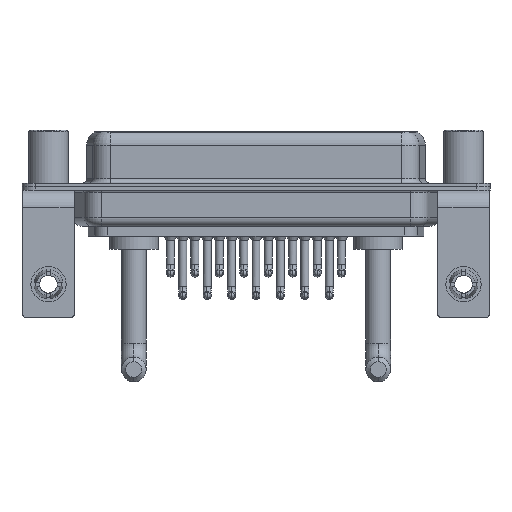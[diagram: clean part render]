
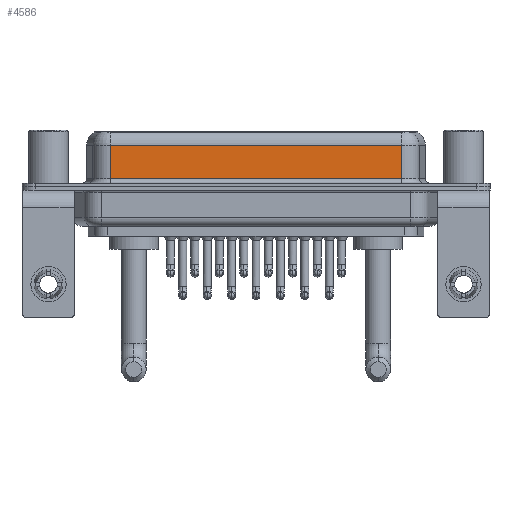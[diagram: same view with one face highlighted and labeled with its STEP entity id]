
A CAD part, front view. The second image highlights one B-rep face of the part: STEP entity #4586.
In plain terms, the highlighted planar face has unit normal (0, -1, 0).
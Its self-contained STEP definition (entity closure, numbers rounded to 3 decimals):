
#231 = VECTOR ( 'NONE', #15734, 1000. ) ;
#411 = LINE ( 'NONE', #7997, #231 ) ;
#575 = LINE ( 'NONE', #22193, #4274 ) ;
#616 = DIRECTION ( 'NONE',  ( 0., 0., -1. ) ) ;
#839 = VERTEX_POINT ( 'NONE', #9190 ) ;
#2372 = VERTEX_POINT ( 'NONE', #9619 ) ;
#2767 = VERTEX_POINT ( 'NONE', #7448 ) ;
#2975 = VECTOR ( 'NONE', #23240, 1000. ) ;
#3736 = CARTESIAN_POINT ( 'NONE',  ( 7.013, -3.95, 0.9 ) ) ;
#3805 = ORIENTED_EDGE ( 'NONE', *, *, #18545, .T. ) ;
#4130 = EDGE_LOOP ( 'NONE', ( #24198, #3805, #7274, #6062 ) ) ;
#4274 = VECTOR ( 'NONE', #20297, 1000. ) ;
#4586 = ADVANCED_FACE ( 'NONE', ( #7038 ), #23507, .F. ) ;
#5246 = EDGE_CURVE ( 'NONE', #10804, #2372, #575, .T. ) ;
#6062 = ORIENTED_EDGE ( 'NONE', *, *, #5246, .T. ) ;
#6183 = LINE ( 'NONE', #21618, #18519 ) ;
#7038 = FACE_OUTER_BOUND ( 'NONE', #4130, .T. ) ;
#7274 = ORIENTED_EDGE ( 'NONE', *, *, #21996, .T. ) ;
#7448 = CARTESIAN_POINT ( 'NONE',  ( 7.013, -3.95, 4.65 ) ) ;
#7997 = CARTESIAN_POINT ( 'NONE',  ( 40.037, -3.95, 4.65 ) ) ;
#8340 = DIRECTION ( 'NONE',  ( 0., 0., 1. ) ) ;
#8921 = CARTESIAN_POINT ( 'NONE',  ( 40.037, -3.95, 6.4 ) ) ;
#9074 = AXIS2_PLACEMENT_3D ( 'NONE', #8921, #12725, #8340 ) ;
#9190 = CARTESIAN_POINT ( 'NONE',  ( 40.037, -3.95, 4.65 ) ) ;
#9619 = CARTESIAN_POINT ( 'NONE',  ( 40.037, -3.95, 0.9 ) ) ;
#10804 = VERTEX_POINT ( 'NONE', #3736 ) ;
#12725 = DIRECTION ( 'NONE',  ( 0., 1., 0. ) ) ;
#14826 = EDGE_CURVE ( 'NONE', #839, #2372, #15296, .T. ) ;
#15296 = LINE ( 'NONE', #15672, #2975 ) ;
#15672 = CARTESIAN_POINT ( 'NONE',  ( 40.037, -3.95, 6.4 ) ) ;
#15734 = DIRECTION ( 'NONE',  ( -1., 0., 0. ) ) ;
#18519 = VECTOR ( 'NONE', #616, 1000. ) ;
#18545 = EDGE_CURVE ( 'NONE', #839, #2767, #411, .T. ) ;
#20297 = DIRECTION ( 'NONE',  ( 1., 0., 0. ) ) ;
#21618 = CARTESIAN_POINT ( 'NONE',  ( 7.013, -3.95, 6.4 ) ) ;
#21996 = EDGE_CURVE ( 'NONE', #2767, #10804, #6183, .T. ) ;
#22193 = CARTESIAN_POINT ( 'NONE',  ( 40.037, -3.95, 0.9 ) ) ;
#23240 = DIRECTION ( 'NONE',  ( 0., 0., -1. ) ) ;
#23507 = PLANE ( 'NONE',  #9074 ) ;
#24198 = ORIENTED_EDGE ( 'NONE', *, *, #14826, .F. ) ;
